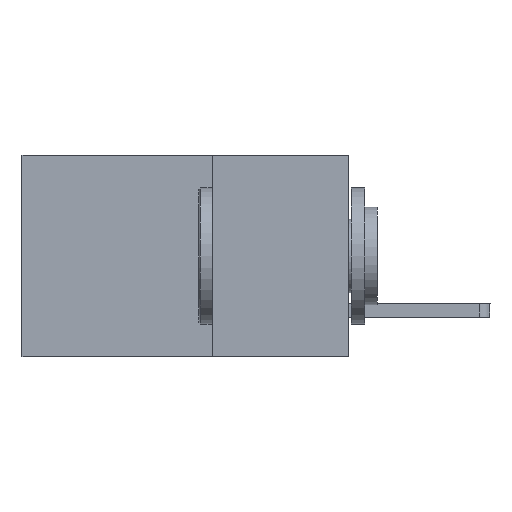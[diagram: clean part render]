
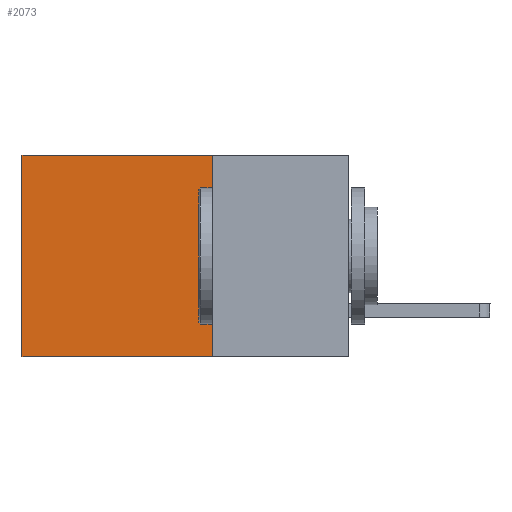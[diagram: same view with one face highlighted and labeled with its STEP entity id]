
A CAD part, left-side view. The second image highlights one B-rep face of the part: STEP entity #2073.
In plain terms, the highlighted planar face has unit normal (-1, 0, 0).
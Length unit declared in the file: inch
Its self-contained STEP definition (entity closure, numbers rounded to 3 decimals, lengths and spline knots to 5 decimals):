
#26 = VECTOR ( 'NONE', #3859, 39.37008 ) ;
#389 = LINE ( 'NONE', #3717, #5608 ) ;
#390 = DIRECTION ( 'NONE',  ( 0., 0., -1. ) ) ;
#988 = DIRECTION ( 'NONE',  ( 0., 0., -1. ) ) ;
#1193 = AXIS2_PLACEMENT_3D ( 'NONE', #5536, #7799, #6137 ) ;
#1221 = EDGE_CURVE ( 'NONE', #3907, #1354, #2732, .T. ) ;
#1354 = VERTEX_POINT ( 'NONE', #2182 ) ;
#2073 = ADVANCED_FACE ( 'NONE', ( #2441 ), #9204, .F. ) ;
#2182 = CARTESIAN_POINT ( 'NONE',  ( 0.2615, 0.6, -0.37 ) ) ;
#2441 = FACE_OUTER_BOUND ( 'NONE', #3184, .T. ) ;
#2582 = CARTESIAN_POINT ( 'NONE',  ( 0.2615, 0.6, 0. ) ) ;
#2732 = LINE ( 'NONE', #3531, #6437 ) ;
#3184 = EDGE_LOOP ( 'NONE', ( #4300, #4140, #5363, #4206 ) ) ;
#3531 = CARTESIAN_POINT ( 'NONE',  ( 0.2615, 0.6, -0.37 ) ) ;
#3717 = CARTESIAN_POINT ( 'NONE',  ( 0.2615, 0.25, -0.37 ) ) ;
#3859 = DIRECTION ( 'NONE',  ( 0., 1., 0. ) ) ;
#3907 = VERTEX_POINT ( 'NONE', #2582 ) ;
#4140 = ORIENTED_EDGE ( 'NONE', *, *, #5121, .F. ) ;
#4206 = ORIENTED_EDGE ( 'NONE', *, *, #4468, .T. ) ;
#4300 = ORIENTED_EDGE ( 'NONE', *, *, #1221, .T. ) ;
#4413 = VERTEX_POINT ( 'NONE', #6845 ) ;
#4468 = EDGE_CURVE ( 'NONE', #4413, #3907, #8364, .T. ) ;
#4469 = DIRECTION ( 'NONE',  ( 0., 1., 0. ) ) ;
#4792 = LINE ( 'NONE', #9438, #5503 ) ;
#4877 = VERTEX_POINT ( 'NONE', #9050 ) ;
#5121 = EDGE_CURVE ( 'NONE', #4877, #1354, #389, .T. ) ;
#5363 = ORIENTED_EDGE ( 'NONE', *, *, #7673, .F. ) ;
#5503 = VECTOR ( 'NONE', #988, 39.37008 ) ;
#5536 = CARTESIAN_POINT ( 'NONE',  ( 0.2615, 0.25, -0.37 ) ) ;
#5608 = VECTOR ( 'NONE', #4469, 39.37008 ) ;
#6137 = DIRECTION ( 'NONE',  ( 0., 0., -1. ) ) ;
#6437 = VECTOR ( 'NONE', #390, 39.37008 ) ;
#6845 = CARTESIAN_POINT ( 'NONE',  ( 0.2615, 0.25, 0. ) ) ;
#7673 = EDGE_CURVE ( 'NONE', #4413, #4877, #4792, .T. ) ;
#7799 = DIRECTION ( 'NONE',  ( 1., 0., 0. ) ) ;
#8364 = LINE ( 'NONE', #9103, #26 ) ;
#9050 = CARTESIAN_POINT ( 'NONE',  ( 0.2615, 0.25, -0.37 ) ) ;
#9103 = CARTESIAN_POINT ( 'NONE',  ( 0.2615, 0.25, 0. ) ) ;
#9204 = PLANE ( 'NONE',  #1193 ) ;
#9438 = CARTESIAN_POINT ( 'NONE',  ( 0.2615, 0.25, -0.37 ) ) ;
